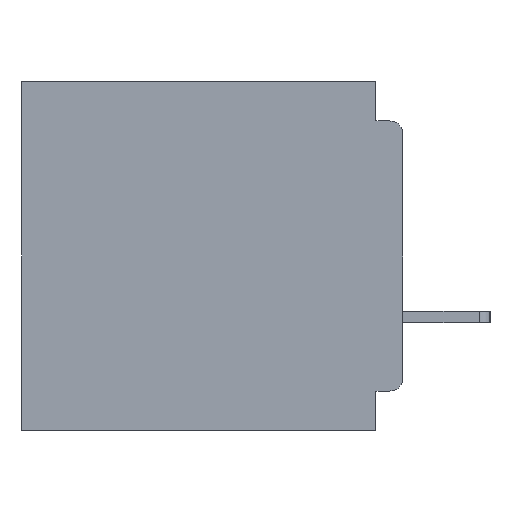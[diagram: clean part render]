
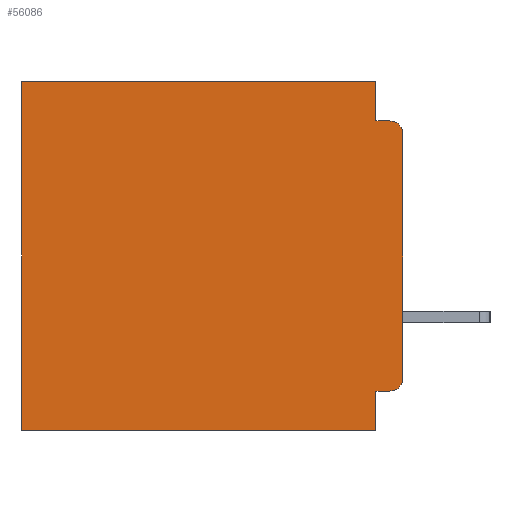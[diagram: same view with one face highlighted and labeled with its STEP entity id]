
A CAD part, left-side view. The second image highlights one B-rep face of the part: STEP entity #56086.
In plain terms, the highlighted planar face has unit normal (-1, 0, 0).
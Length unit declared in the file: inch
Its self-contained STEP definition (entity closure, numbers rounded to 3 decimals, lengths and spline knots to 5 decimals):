
#143 = CARTESIAN_POINT ( 'NONE',  ( 0.3, 0.031, 0. ) ) ;
#846 = ORIENTED_EDGE ( 'NONE', *, *, #50845, .F. ) ;
#1123 = VERTEX_POINT ( 'NONE', #51393 ) ;
#1170 = DIRECTION ( 'NONE',  ( -1., 0., 0. ) ) ;
#1821 = CARTESIAN_POINT ( 'NONE',  ( 0.3, 0., -0.4 ) ) ;
#2838 = LINE ( 'NONE', #12623, #23346 ) ;
#2853 = EDGE_CURVE ( 'NONE', #53187, #1123, #4559, .T. ) ;
#3214 = CIRCLE ( 'NONE', #32587, 0.015 ) ;
#4090 = LINE ( 'NONE', #46029, #52400 ) ;
#4559 = LINE ( 'NONE', #1821, #28000 ) ;
#4744 = VECTOR ( 'NONE', #32486, 39.37008 ) ;
#5373 = VERTEX_POINT ( 'NONE', #143 ) ;
#5746 = VERTEX_POINT ( 'NONE', #40517 ) ;
#8075 = VECTOR ( 'NONE', #60367, 39.37008 ) ;
#11536 = VERTEX_POINT ( 'NONE', #31505 ) ;
#11797 = DIRECTION ( 'NONE',  ( 0., 0., -1. ) ) ;
#12320 = AXIS2_PLACEMENT_3D ( 'NONE', #29256, #1170, #33981 ) ;
#12623 = CARTESIAN_POINT ( 'NONE',  ( 0.3, 0., 0. ) ) ;
#12709 = ORIENTED_EDGE ( 'NONE', *, *, #52739, .T. ) ;
#13287 = DIRECTION ( 'NONE',  ( 0., 0., -1. ) ) ;
#13370 = DIRECTION ( 'NONE',  ( -1., 0., 0. ) ) ;
#14416 = CARTESIAN_POINT ( 'NONE',  ( 0.3, 0., -0.4 ) ) ;
#16451 = VECTOR ( 'NONE', #17860, 39.37008 ) ;
#17860 = DIRECTION ( 'NONE',  ( 0., 1., 0. ) ) ;
#17913 = CARTESIAN_POINT ( 'NONE',  ( 0.3, 0., -0.06 ) ) ;
#17922 = LINE ( 'NONE', #31853, #16451 ) ;
#20377 = VERTEX_POINT ( 'NONE', #34058 ) ;
#20475 = LINE ( 'NONE', #41635, #8075 ) ;
#21097 = EDGE_CURVE ( 'NONE', #57155, #20377, #49844, .T. ) ;
#21285 = ORIENTED_EDGE ( 'NONE', *, *, #21097, .F. ) ;
#21546 = EDGE_CURVE ( 'NONE', #23826, #20377, #20475, .T. ) ;
#22203 = EDGE_LOOP ( 'NONE', ( #37070, #59539, #846, #58739, #45522, #35041, #21285, #54957, #32487, #12709 ) ) ;
#23346 = VECTOR ( 'NONE', #49843, 39.37008 ) ;
#23826 = VERTEX_POINT ( 'NONE', #46677 ) ;
#27273 = CARTESIAN_POINT ( 'NONE',  ( 0.3, 0.015, -0.355 ) ) ;
#28000 = VECTOR ( 'NONE', #41287, 39.37008 ) ;
#28420 = CIRCLE ( 'NONE', #12320, 0.015 ) ;
#29256 = CARTESIAN_POINT ( 'NONE',  ( 0.3, 0.015, -0.34 ) ) ;
#29961 = CARTESIAN_POINT ( 'NONE',  ( 0.3, 0.031, -0.4 ) ) ;
#29979 = CARTESIAN_POINT ( 'NONE',  ( 0.3, 0.031, -0.045 ) ) ;
#30706 = DIRECTION ( 'NONE',  ( 0., 0., -1. ) ) ;
#31505 = CARTESIAN_POINT ( 'NONE',  ( 0.3, 0.031, -0.355 ) ) ;
#31853 = CARTESIAN_POINT ( 'NONE',  ( 0.3, 0., -0.355 ) ) ;
#32487 = ORIENTED_EDGE ( 'NONE', *, *, #39771, .F. ) ;
#32486 = DIRECTION ( 'NONE',  ( 0., -1., 0. ) ) ;
#32587 = AXIS2_PLACEMENT_3D ( 'NONE', #41446, #13370, #46108 ) ;
#33710 = FACE_OUTER_BOUND ( 'NONE', #22203, .T. ) ;
#33981 = DIRECTION ( 'NONE',  ( 0., 0., -1. ) ) ;
#34058 = CARTESIAN_POINT ( 'NONE',  ( 0.3, 0.437, -0.4 ) ) ;
#35041 = ORIENTED_EDGE ( 'NONE', *, *, #21546, .T. ) ;
#35211 = CARTESIAN_POINT ( 'NONE',  ( 0.3, 0., -0.4 ) ) ;
#36833 = LINE ( 'NONE', #48849, #60174 ) ;
#37070 = ORIENTED_EDGE ( 'NONE', *, *, #2853, .F. ) ;
#38458 = VERTEX_POINT ( 'NONE', #27273 ) ;
#39771 = EDGE_CURVE ( 'NONE', #38458, #11536, #17922, .T. ) ;
#40517 = CARTESIAN_POINT ( 'NONE',  ( 0.3, 0.015, -0.045 ) ) ;
#41287 = DIRECTION ( 'NONE',  ( 0., 0., -1. ) ) ;
#41446 = CARTESIAN_POINT ( 'NONE',  ( 0.3, 0.015, -0.06 ) ) ;
#41635 = CARTESIAN_POINT ( 'NONE',  ( 0.3, 0.437, -0.4 ) ) ;
#42674 = VERTEX_POINT ( 'NONE', #29979 ) ;
#45024 = LINE ( 'NONE', #46354, #4744 ) ;
#45522 = ORIENTED_EDGE ( 'NONE', *, *, #56689, .T. ) ;
#46029 = CARTESIAN_POINT ( 'NONE',  ( 0.3, 0.031, 0. ) ) ;
#46108 = DIRECTION ( 'NONE',  ( 0., 0., -1. ) ) ;
#46354 = CARTESIAN_POINT ( 'NONE',  ( 0.3, 0., -0.045 ) ) ;
#46677 = CARTESIAN_POINT ( 'NONE',  ( 0.3, 0.437, 0. ) ) ;
#48391 = VECTOR ( 'NONE', #51872, 39.37008 ) ;
#48849 = CARTESIAN_POINT ( 'NONE',  ( 0.3, 0.031, -0.4 ) ) ;
#49843 = DIRECTION ( 'NONE',  ( 0., 1., 0. ) ) ;
#49844 = LINE ( 'NONE', #14416, #48391 ) ;
#50154 = EDGE_CURVE ( 'NONE', #5373, #42674, #4090, .T. ) ;
#50845 = EDGE_CURVE ( 'NONE', #42674, #5746, #45024, .T. ) ;
#51393 = CARTESIAN_POINT ( 'NONE',  ( 0.3, 0., -0.34 ) ) ;
#51872 = DIRECTION ( 'NONE',  ( 0., 1., 0. ) ) ;
#52400 = VECTOR ( 'NONE', #13287, 39.37008 ) ;
#52739 = EDGE_CURVE ( 'NONE', #38458, #1123, #28420, .T. ) ;
#53187 = VERTEX_POINT ( 'NONE', #17913 ) ;
#54007 = PLANE ( 'NONE',  #55956 ) ;
#54807 = EDGE_CURVE ( 'NONE', #11536, #57155, #36833, .T. ) ;
#54957 = ORIENTED_EDGE ( 'NONE', *, *, #54807, .F. ) ;
#55956 = AXIS2_PLACEMENT_3D ( 'NONE', #35211, #58681, #30706 ) ;
#56086 = ADVANCED_FACE ( 'NONE', ( #33710 ), #54007, .F. ) ;
#56689 = EDGE_CURVE ( 'NONE', #5373, #23826, #2838, .T. ) ;
#57155 = VERTEX_POINT ( 'NONE', #29961 ) ;
#58681 = DIRECTION ( 'NONE',  ( 1., 0., 0. ) ) ;
#58739 = ORIENTED_EDGE ( 'NONE', *, *, #50154, .F. ) ;
#59434 = EDGE_CURVE ( 'NONE', #53187, #5746, #3214, .T. ) ;
#59539 = ORIENTED_EDGE ( 'NONE', *, *, #59434, .T. ) ;
#60174 = VECTOR ( 'NONE', #11797, 39.37008 ) ;
#60367 = DIRECTION ( 'NONE',  ( 0., 0., -1. ) ) ;
